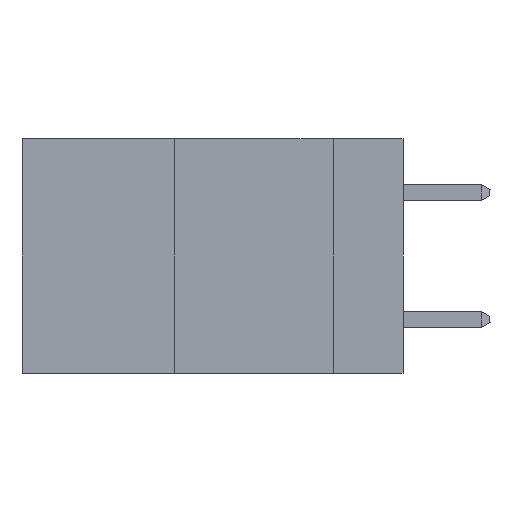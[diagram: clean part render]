
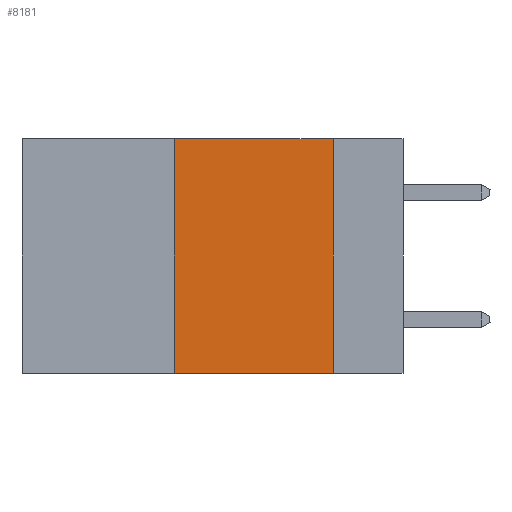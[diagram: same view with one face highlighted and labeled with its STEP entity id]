
A CAD part, left-side view. The second image highlights one B-rep face of the part: STEP entity #8181.
In plain terms, the highlighted planar face has unit normal (-1, 0, 0).
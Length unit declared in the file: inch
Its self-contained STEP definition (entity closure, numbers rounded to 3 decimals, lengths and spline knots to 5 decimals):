
#207 = VERTEX_POINT ( 'NONE', #11299 ) ;
#2364 = CARTESIAN_POINT ( 'NONE',  ( 0., 0.11, 0. ) ) ;
#2467 = AXIS2_PLACEMENT_3D ( 'NONE', #11486, #5281, #13970 ) ;
#2683 = PLANE ( 'NONE',  #2467 ) ;
#2783 = DIRECTION ( 'NONE',  ( 0., -1., 0. ) ) ;
#2835 = VECTOR ( 'NONE', #4238, 39.37008 ) ;
#3103 = ORIENTED_EDGE ( 'NONE', *, *, #6113, .F. ) ;
#3885 = CARTESIAN_POINT ( 'NONE',  ( 0., 0.36, 0. ) ) ;
#4223 = CARTESIAN_POINT ( 'NONE',  ( 0., 0.6, 0. ) ) ;
#4238 = DIRECTION ( 'NONE',  ( 0., 0., 1. ) ) ;
#5281 = DIRECTION ( 'NONE',  ( 1., 0., 0. ) ) ;
#5651 = LINE ( 'NONE', #4223, #6436 ) ;
#6113 = EDGE_CURVE ( 'NONE', #207, #14079, #15593, .T. ) ;
#6136 = VECTOR ( 'NONE', #9945, 39.37008 ) ;
#6436 = VECTOR ( 'NONE', #15433, 39.37008 ) ;
#6470 = CARTESIAN_POINT ( 'NONE',  ( 0., 0.11, -0.37 ) ) ;
#7255 = VERTEX_POINT ( 'NONE', #12209 ) ;
#7314 = ORIENTED_EDGE ( 'NONE', *, *, #11616, .T. ) ;
#7462 = VERTEX_POINT ( 'NONE', #3885 ) ;
#8181 = ADVANCED_FACE ( 'NONE', ( #8950 ), #2683, .F. ) ;
#8950 = FACE_OUTER_BOUND ( 'NONE', #10257, .T. ) ;
#9046 = LINE ( 'NONE', #10340, #9447 ) ;
#9447 = VECTOR ( 'NONE', #2783, 39.37008 ) ;
#9945 = DIRECTION ( 'NONE',  ( 0., 0., -1. ) ) ;
#10216 = ORIENTED_EDGE ( 'NONE', *, *, #13598, .F. ) ;
#10257 = EDGE_LOOP ( 'NONE', ( #3103, #13595, #10216, #7314 ) ) ;
#10340 = CARTESIAN_POINT ( 'NONE',  ( 0., 0.6, -0.37 ) ) ;
#11299 = CARTESIAN_POINT ( 'NONE',  ( 0., 0.11, 0. ) ) ;
#11486 = CARTESIAN_POINT ( 'NONE',  ( 0., 0.6, 0. ) ) ;
#11616 = EDGE_CURVE ( 'NONE', #7255, #14079, #9046, .T. ) ;
#12209 = CARTESIAN_POINT ( 'NONE',  ( 0., 0.36, -0.37 ) ) ;
#13595 = ORIENTED_EDGE ( 'NONE', *, *, #14630, .F. ) ;
#13598 = EDGE_CURVE ( 'NONE', #7255, #7462, #15720, .T. ) ;
#13970 = DIRECTION ( 'NONE',  ( 0., 0., -1. ) ) ;
#14079 = VERTEX_POINT ( 'NONE', #6470 ) ;
#14230 = CARTESIAN_POINT ( 'NONE',  ( 0., 0.36, 0. ) ) ;
#14630 = EDGE_CURVE ( 'NONE', #7462, #207, #5651, .T. ) ;
#15433 = DIRECTION ( 'NONE',  ( 0., -1., 0. ) ) ;
#15593 = LINE ( 'NONE', #2364, #6136 ) ;
#15720 = LINE ( 'NONE', #14230, #2835 ) ;
